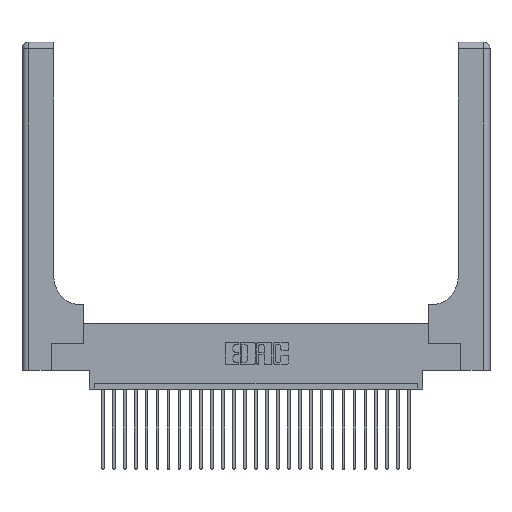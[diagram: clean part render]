
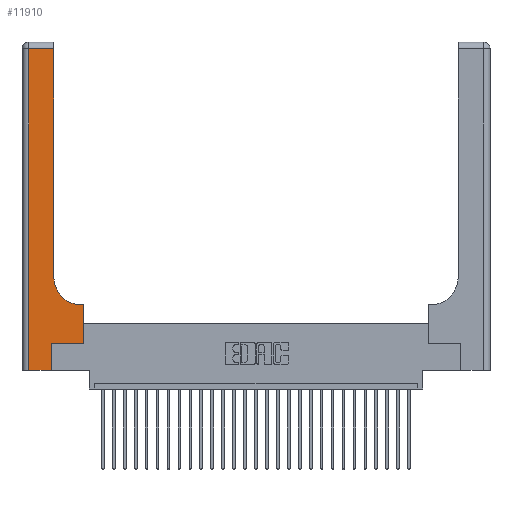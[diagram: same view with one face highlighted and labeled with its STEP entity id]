
A CAD part, top view. The second image highlights one B-rep face of the part: STEP entity #11910.
In plain terms, the highlighted planar face has unit normal (0, 0, 1).
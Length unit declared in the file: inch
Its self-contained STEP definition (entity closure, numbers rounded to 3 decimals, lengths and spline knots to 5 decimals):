
#763 = EDGE_CURVE ( 'NONE', #25771, #19575, #16242, .T. ) ;
#886 = DIRECTION ( 'NONE',  ( -1., 0., 0. ) ) ;
#1085 = DIRECTION ( 'NONE',  ( 1., 0., 0. ) ) ;
#1091 = VERTEX_POINT ( 'NONE', #27340 ) ;
#1215 = VERTEX_POINT ( 'NONE', #6014 ) ;
#1921 = VECTOR ( 'NONE', #5254, 39.37008 ) ;
#2918 = VECTOR ( 'NONE', #16847, 39.37008 ) ;
#3191 = CARTESIAN_POINT ( 'NONE',  ( 0.5415, 0.85, 0.37 ) ) ;
#3492 = VECTOR ( 'NONE', #4135, 39.37008 ) ;
#3642 = AXIS2_PLACEMENT_3D ( 'NONE', #20769, #24800, #11388 ) ;
#3702 = LINE ( 'NONE', #9073, #21529 ) ;
#4135 = DIRECTION ( 'NONE',  ( 0., 1., 0. ) ) ;
#4888 = CARTESIAN_POINT ( 'NONE',  ( 0.2915, 0.85, 0.37 ) ) ;
#5254 = DIRECTION ( 'NONE',  ( 1., 0., 0. ) ) ;
#6014 = CARTESIAN_POINT ( 'NONE',  ( 0.5415, 0.6, 0.37 ) ) ;
#6089 = CARTESIAN_POINT ( 'NONE',  ( 0.5585, 0.25, 0.37 ) ) ;
#7435 = ORIENTED_EDGE ( 'NONE', *, *, #11336, .T. ) ;
#8035 = DIRECTION ( 'NONE',  ( -1., 0., 0. ) ) ;
#8396 = LINE ( 'NONE', #17193, #3492 ) ;
#9073 = CARTESIAN_POINT ( 'NONE',  ( 0.06, 3., 0.37 ) ) ;
#10094 = LINE ( 'NONE', #21596, #23435 ) ;
#10205 = AXIS2_PLACEMENT_3D ( 'NONE', #3191, #18830, #1085 ) ;
#10267 = ORIENTED_EDGE ( 'NONE', *, *, #16181, .T. ) ;
#10873 = VERTEX_POINT ( 'NONE', #4888 ) ;
#11336 = EDGE_CURVE ( 'NONE', #1091, #25771, #14055, .T. ) ;
#11388 = DIRECTION ( 'NONE',  ( -1., 0., 0. ) ) ;
#11910 = ADVANCED_FACE ( 'NONE', ( #16821 ), #18518, .F. ) ;
#13078 = DIRECTION ( 'NONE',  ( 1., 0., 0. ) ) ;
#14041 = EDGE_CURVE ( 'NONE', #27192, #21055, #3702, .T. ) ;
#14055 = LINE ( 'NONE', #19027, #2918 ) ;
#14203 = EDGE_CURVE ( 'NONE', #1215, #10873, #25034, .T. ) ;
#14380 = LINE ( 'NONE', #16250, #19351 ) ;
#15084 = VERTEX_POINT ( 'NONE', #24892 ) ;
#15809 = EDGE_LOOP ( 'NONE', ( #23880, #23592, #26932, #19659, #7435, #27861, #10267, #16560, #19137 ) ) ;
#16181 = EDGE_CURVE ( 'NONE', #19575, #15084, #28121, .T. ) ;
#16242 = LINE ( 'NONE', #26592, #19094 ) ;
#16250 = CARTESIAN_POINT ( 'NONE',  ( 0.2915, 0.6, 0.37 ) ) ;
#16560 = ORIENTED_EDGE ( 'NONE', *, *, #22272, .T. ) ;
#16606 = EDGE_CURVE ( 'NONE', #21055, #1091, #27059, .T. ) ;
#16821 = FACE_OUTER_BOUND ( 'NONE', #15809, .T. ) ;
#16847 = DIRECTION ( 'NONE',  ( 0., 1., 0. ) ) ;
#17193 = CARTESIAN_POINT ( 'NONE',  ( 0.2915, 3., 0.37 ) ) ;
#17841 = VERTEX_POINT ( 'NONE', #23639 ) ;
#17966 = DIRECTION ( 'NONE',  ( 0., 1., 0. ) ) ;
#18361 = EDGE_CURVE ( 'NONE', #17841, #27192, #10094, .T. ) ;
#18518 = PLANE ( 'NONE',  #3642 ) ;
#18645 = VECTOR ( 'NONE', #17966, 39.37008 ) ;
#18830 = DIRECTION ( 'NONE',  ( 0., 0., -1. ) ) ;
#19027 = CARTESIAN_POINT ( 'NONE',  ( 0.269, 0., 0.37 ) ) ;
#19094 = VECTOR ( 'NONE', #13078, 39.37008 ) ;
#19137 = ORIENTED_EDGE ( 'NONE', *, *, #14203, .T. ) ;
#19351 = VECTOR ( 'NONE', #886, 39.37008 ) ;
#19575 = VERTEX_POINT ( 'NONE', #6089 ) ;
#19659 = ORIENTED_EDGE ( 'NONE', *, *, #16606, .T. ) ;
#19684 = CARTESIAN_POINT ( 'NONE',  ( 0.06, 0., 0.37 ) ) ;
#20323 = DIRECTION ( 'NONE',  ( 0., -1., 0. ) ) ;
#20769 = CARTESIAN_POINT ( 'NONE',  ( 0., 3., 0.37 ) ) ;
#21055 = VERTEX_POINT ( 'NONE', #19684 ) ;
#21529 = VECTOR ( 'NONE', #20323, 39.37008 ) ;
#21596 = CARTESIAN_POINT ( 'NONE',  ( 0., 2.94, 0.37 ) ) ;
#22272 = EDGE_CURVE ( 'NONE', #15084, #1215, #14380, .T. ) ;
#23240 = CARTESIAN_POINT ( 'NONE',  ( 0., 0., 0.37 ) ) ;
#23435 = VECTOR ( 'NONE', #8035, 39.37008 ) ;
#23592 = ORIENTED_EDGE ( 'NONE', *, *, #18361, .T. ) ;
#23639 = CARTESIAN_POINT ( 'NONE',  ( 0.2915, 2.94, 0.37 ) ) ;
#23880 = ORIENTED_EDGE ( 'NONE', *, *, #24011, .T. ) ;
#23907 = CARTESIAN_POINT ( 'NONE',  ( 0.5585, 0.25, 0.37 ) ) ;
#24011 = EDGE_CURVE ( 'NONE', #10873, #17841, #8396, .T. ) ;
#24800 = DIRECTION ( 'NONE',  ( 0., 0., -1. ) ) ;
#24892 = CARTESIAN_POINT ( 'NONE',  ( 0.5585, 0.6, 0.37 ) ) ;
#25034 = CIRCLE ( 'NONE', #10205, 0.25 ) ;
#25771 = VERTEX_POINT ( 'NONE', #26133 ) ;
#26133 = CARTESIAN_POINT ( 'NONE',  ( 0.269, 0.25, 0.37 ) ) ;
#26592 = CARTESIAN_POINT ( 'NONE',  ( 0.269, 0.25, 0.37 ) ) ;
#26932 = ORIENTED_EDGE ( 'NONE', *, *, #14041, .T. ) ;
#27059 = LINE ( 'NONE', #23240, #1921 ) ;
#27192 = VERTEX_POINT ( 'NONE', #28110 ) ;
#27340 = CARTESIAN_POINT ( 'NONE',  ( 0.269, 0., 0.37 ) ) ;
#27861 = ORIENTED_EDGE ( 'NONE', *, *, #763, .T. ) ;
#28110 = CARTESIAN_POINT ( 'NONE',  ( 0.06, 2.94, 0.37 ) ) ;
#28121 = LINE ( 'NONE', #23907, #18645 ) ;
